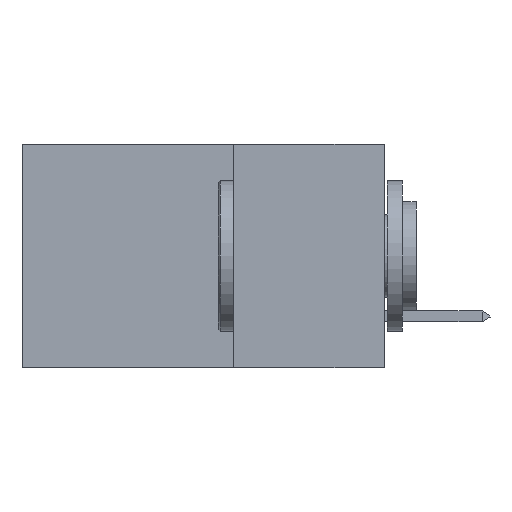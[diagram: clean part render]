
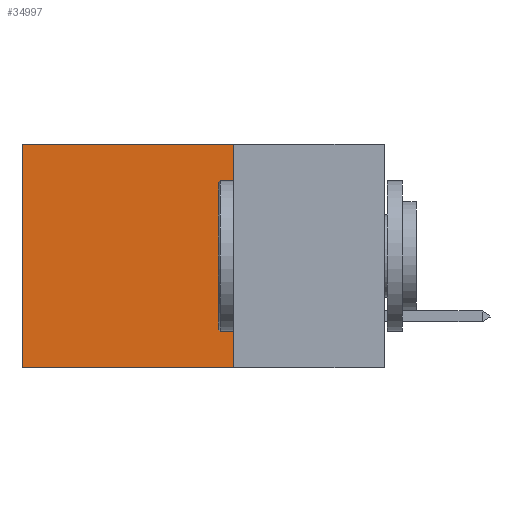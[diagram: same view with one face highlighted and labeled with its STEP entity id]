
A CAD part, left-side view. The second image highlights one B-rep face of the part: STEP entity #34997.
In plain terms, the highlighted planar face has unit normal (-1, 0, 0).
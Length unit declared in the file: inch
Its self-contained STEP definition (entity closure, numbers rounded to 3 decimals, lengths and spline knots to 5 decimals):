
#677 = VECTOR ( 'NONE', #37314, 39.37008 ) ;
#834 = DIRECTION ( 'NONE',  ( 1., 0., 0. ) ) ;
#1233 = CARTESIAN_POINT ( 'NONE',  ( 0.2875, 0.25, -0.37 ) ) ;
#1253 = EDGE_CURVE ( 'NONE', #1938, #5063, #22399, .T. ) ;
#1938 = VERTEX_POINT ( 'NONE', #34342 ) ;
#4596 = ORIENTED_EDGE ( 'NONE', *, *, #30806, .T. ) ;
#5063 = VERTEX_POINT ( 'NONE', #39875 ) ;
#9674 = DIRECTION ( 'NONE',  ( 0., 0., -1. ) ) ;
#10558 = VERTEX_POINT ( 'NONE', #38744 ) ;
#11537 = VECTOR ( 'NONE', #41951, 39.37008 ) ;
#12120 = VECTOR ( 'NONE', #9674, 39.37008 ) ;
#12588 = ORIENTED_EDGE ( 'NONE', *, *, #36529, .F. ) ;
#12609 = VECTOR ( 'NONE', #44255, 39.37008 ) ;
#18018 = PLANE ( 'NONE',  #21172 ) ;
#21172 = AXIS2_PLACEMENT_3D ( 'NONE', #35346, #834, #30393 ) ;
#21241 = CARTESIAN_POINT ( 'NONE',  ( 0.2875, 0.25, 0. ) ) ;
#21255 = LINE ( 'NONE', #36050, #677 ) ;
#22399 = LINE ( 'NONE', #21241, #12120 ) ;
#25686 = CARTESIAN_POINT ( 'NONE',  ( 0.2875, 0.6, 0. ) ) ;
#30393 = DIRECTION ( 'NONE',  ( 0., 0., -1. ) ) ;
#30551 = VERTEX_POINT ( 'NONE', #25686 ) ;
#30806 = EDGE_CURVE ( 'NONE', #1938, #30551, #45169, .T. ) ;
#33999 = EDGE_CURVE ( 'NONE', #30551, #10558, #21255, .T. ) ;
#34342 = CARTESIAN_POINT ( 'NONE',  ( 0.2875, 0.25, 0. ) ) ;
#34997 = ADVANCED_FACE ( 'NONE', ( #46876 ), #18018, .F. ) ;
#35346 = CARTESIAN_POINT ( 'NONE',  ( 0.2875, 0.25, 0. ) ) ;
#36050 = CARTESIAN_POINT ( 'NONE',  ( 0.2875, 0.6, 0. ) ) ;
#36529 = EDGE_CURVE ( 'NONE', #5063, #10558, #47365, .T. ) ;
#37314 = DIRECTION ( 'NONE',  ( 0., 0., -1. ) ) ;
#38498 = ORIENTED_EDGE ( 'NONE', *, *, #33999, .T. ) ;
#38744 = CARTESIAN_POINT ( 'NONE',  ( 0.2875, 0.6, -0.37 ) ) ;
#39875 = CARTESIAN_POINT ( 'NONE',  ( 0.2875, 0.25, -0.37 ) ) ;
#41951 = DIRECTION ( 'NONE',  ( 0., 1., 0. ) ) ;
#44255 = DIRECTION ( 'NONE',  ( 0., 1., 0. ) ) ;
#45169 = LINE ( 'NONE', #46417, #11537 ) ;
#46417 = CARTESIAN_POINT ( 'NONE',  ( 0.2875, 0.25, 0. ) ) ;
#46876 = FACE_OUTER_BOUND ( 'NONE', #48276, .T. ) ;
#47365 = LINE ( 'NONE', #1233, #12609 ) ;
#48276 = EDGE_LOOP ( 'NONE', ( #38498, #12588, #48609, #4596 ) ) ;
#48609 = ORIENTED_EDGE ( 'NONE', *, *, #1253, .F. ) ;
